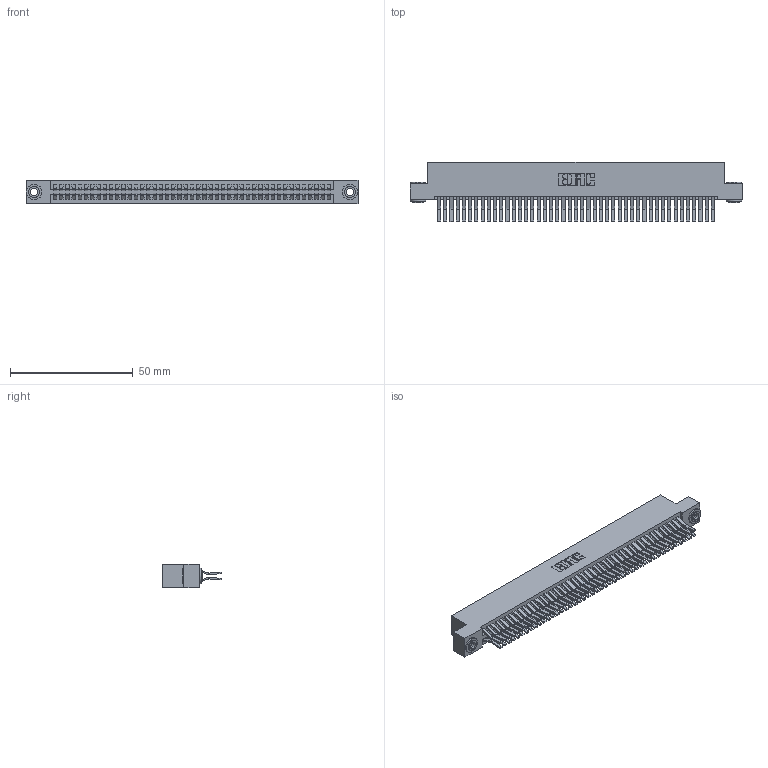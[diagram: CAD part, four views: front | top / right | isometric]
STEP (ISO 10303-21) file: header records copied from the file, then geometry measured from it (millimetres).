
FILE_DESCRIPTION (( 'STEP AP203' ), '1' );
FILE_NAME ('345-090-560-203.STEP', '2019-11-01T17:38:55', ( '' ), ( '' ), 'SwSTEP 2.0', 'SolidWorks 2016', '' );
FILE_SCHEMA (( 'CONFIG_CONTROL_DESIGN' ));
Length unit declared in the file: inch
Products named in the file (4): 345-090-560-203; 345-250-002_345-250-002-102; 345 Part_Flush Mounting Lugs - 0.156 Dia-TH; 345-292-001_560 Tail
Assembly tree (93 placements, depth 2):
  345-090-560-203
    345 Part_Flush Mounting Lugs - 0.156 Dia-TH
    345-292-001_560 Tail  x90
    345-250-002_345-250-002-102  x2
Bounding box: 135.51 x 24.45 x 9.4 mm (x, y, z)
Volume: 13800.6 mm3; surface area: 22179.9 mm2
Topology: 93 solids, 93 shells, 4844 faces, 14367 edges, 9454 vertices
Faces by surface type: plane 3060, cylinder 1776, cone 8
Entity records: 35642 total; most frequent: CARTESIAN_POINT 5947, ORIENTED_EDGE 5874, DIRECTION 5275, EDGE_CURVE 2937, VECTOR 2597, LINE 2597, VERTEX_POINT 1954, AXIS2_PLACEMENT_3D 1339
